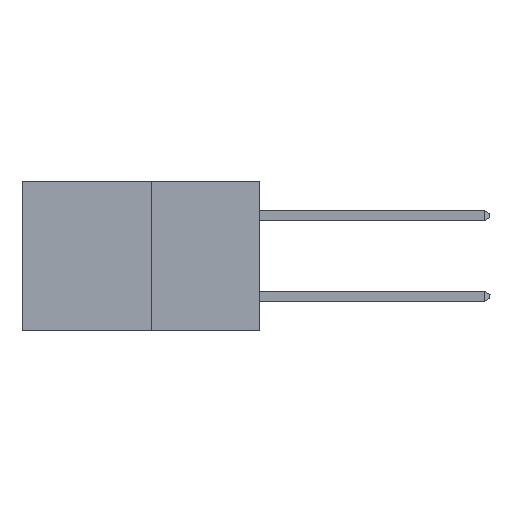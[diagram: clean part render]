
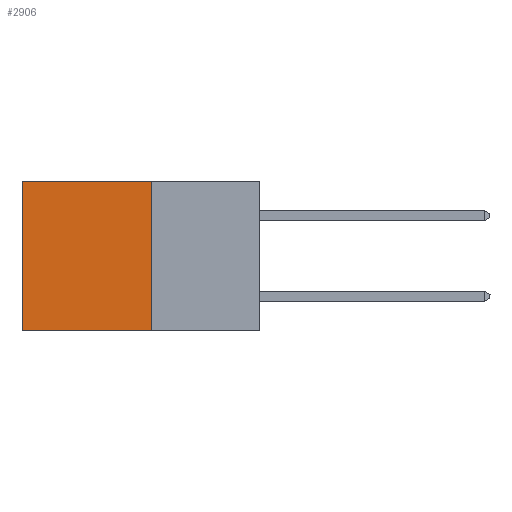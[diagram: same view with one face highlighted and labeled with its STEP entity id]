
A CAD part, left-side view. The second image highlights one B-rep face of the part: STEP entity #2906.
In plain terms, the highlighted planar face has unit normal (-1, 0, 0).
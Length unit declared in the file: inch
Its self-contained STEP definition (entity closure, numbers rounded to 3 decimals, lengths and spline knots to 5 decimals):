
#79 = VERTEX_POINT ( 'NONE', #7774 ) ;
#101 = EDGE_CURVE ( 'NONE', #79, #1484, #4726, .T. ) ;
#133 = LINE ( 'NONE', #2934, #9197 ) ;
#325 = DIRECTION ( 'NONE',  ( 1., 0., 0. ) ) ;
#806 = DIRECTION ( 'NONE',  ( 0., 0., -1. ) ) ;
#1240 = DIRECTION ( 'NONE',  ( 0., 0., -1. ) ) ;
#1484 = VERTEX_POINT ( 'NONE', #3493 ) ;
#1881 = CARTESIAN_POINT ( 'NONE',  ( 0.277, 0.59, -0.37 ) ) ;
#2131 = CARTESIAN_POINT ( 'NONE',  ( 0.277, 0.27, -0.37 ) ) ;
#2643 = CARTESIAN_POINT ( 'NONE',  ( 0.277, 0.27, -0.37 ) ) ;
#2688 = VECTOR ( 'NONE', #5713, 39.37008 ) ;
#2906 = ADVANCED_FACE ( 'NONE', ( #4420 ), #5274, .F. ) ;
#2934 = CARTESIAN_POINT ( 'NONE',  ( 0.277, 0.27, -0.37 ) ) ;
#3282 = EDGE_LOOP ( 'NONE', ( #10471, #5043, #9413, #4764 ) ) ;
#3493 = CARTESIAN_POINT ( 'NONE',  ( 0.277, 0.59, 0. ) ) ;
#3667 = VERTEX_POINT ( 'NONE', #2131 ) ;
#4281 = EDGE_CURVE ( 'NONE', #3667, #9164, #133, .T. ) ;
#4420 = FACE_OUTER_BOUND ( 'NONE', #3282, .T. ) ;
#4726 = LINE ( 'NONE', #5766, #2688 ) ;
#4764 = ORIENTED_EDGE ( 'NONE', *, *, #101, .T. ) ;
#5043 = ORIENTED_EDGE ( 'NONE', *, *, #4281, .F. ) ;
#5274 = PLANE ( 'NONE',  #10040 ) ;
#5594 = EDGE_CURVE ( 'NONE', #1484, #9164, #10865, .T. ) ;
#5713 = DIRECTION ( 'NONE',  ( 0., 1., 0. ) ) ;
#5766 = CARTESIAN_POINT ( 'NONE',  ( 0.277, 0.27, 0. ) ) ;
#5987 = LINE ( 'NONE', #6847, #10002 ) ;
#6535 = VECTOR ( 'NONE', #1240, 39.37008 ) ;
#6610 = DIRECTION ( 'NONE',  ( 0., 0., -1. ) ) ;
#6615 = EDGE_CURVE ( 'NONE', #79, #3667, #5987, .T. ) ;
#6847 = CARTESIAN_POINT ( 'NONE',  ( 0.277, 0.27, -0.37 ) ) ;
#7082 = DIRECTION ( 'NONE',  ( 0., 1., 0. ) ) ;
#7774 = CARTESIAN_POINT ( 'NONE',  ( 0.277, 0.27, 0. ) ) ;
#9164 = VERTEX_POINT ( 'NONE', #1881 ) ;
#9197 = VECTOR ( 'NONE', #7082, 39.37008 ) ;
#9413 = ORIENTED_EDGE ( 'NONE', *, *, #6615, .F. ) ;
#9599 = CARTESIAN_POINT ( 'NONE',  ( 0.277, 0.59, -0.37 ) ) ;
#10002 = VECTOR ( 'NONE', #806, 39.37008 ) ;
#10040 = AXIS2_PLACEMENT_3D ( 'NONE', #2643, #325, #6610 ) ;
#10471 = ORIENTED_EDGE ( 'NONE', *, *, #5594, .T. ) ;
#10865 = LINE ( 'NONE', #9599, #6535 ) ;
